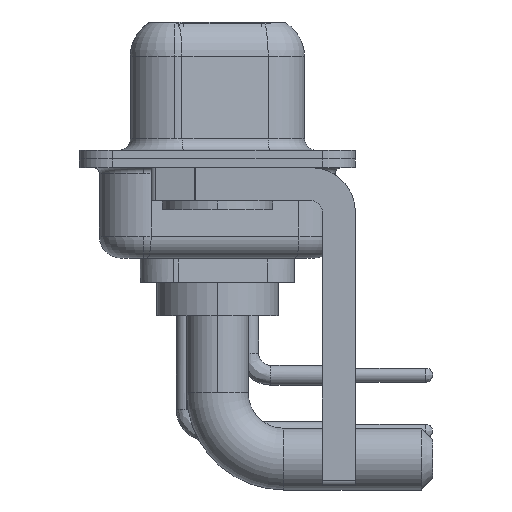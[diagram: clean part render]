
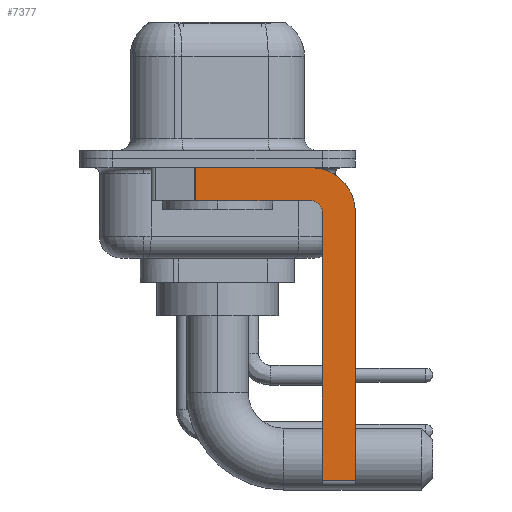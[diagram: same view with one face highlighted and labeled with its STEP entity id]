
A CAD part, left-side view. The second image highlights one B-rep face of the part: STEP entity #7377.
In plain terms, the highlighted planar face has unit normal (-1, 0, 0).
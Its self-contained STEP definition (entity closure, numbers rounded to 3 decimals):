
#596 = CIRCLE ( 'NONE', #11377, 0.5 ) ;
#609 = LINE ( 'NONE', #10292, #14014 ) ;
#762 = CARTESIAN_POINT ( 'NONE',  ( -2.9, -4.75, -2.4 ) ) ;
#1250 = CARTESIAN_POINT ( 'NONE',  ( -2.9, -4.25, -1.9 ) ) ;
#1425 = EDGE_CURVE ( 'NONE', #2869, #2047, #6243, .T. ) ;
#1938 = EDGE_CURVE ( 'NONE', #14677, #5587, #12662, .T. ) ;
#2047 = VERTEX_POINT ( 'NONE', #6836 ) ;
#2358 = EDGE_CURVE ( 'NONE', #2387, #14966, #5190, .T. ) ;
#2387 = VERTEX_POINT ( 'NONE', #14862 ) ;
#2869 = VERTEX_POINT ( 'NONE', #4990 ) ;
#3490 = EDGE_CURVE ( 'NONE', #2387, #14677, #17820, .T. ) ;
#3583 = EDGE_LOOP ( 'NONE', ( #13908, #8388, #13151, #5882, #15429, #6358, #17885, #15256 ) ) ;
#3808 = DIRECTION ( 'NONE',  ( 0., 0., 1. ) ) ;
#3945 = VECTOR ( 'NONE', #9134, 1000. ) ;
#4218 = EDGE_CURVE ( 'NONE', #5587, #2047, #9379, .T. ) ;
#4708 = VECTOR ( 'NONE', #3808, 1000. ) ;
#4990 = CARTESIAN_POINT ( 'NONE',  ( -2.9, -4.75, -14.55 ) ) ;
#5190 = LINE ( 'NONE', #15040, #3945 ) ;
#5485 = DIRECTION ( 'NONE',  ( 0., 0., -1. ) ) ;
#5587 = VERTEX_POINT ( 'NONE', #12764 ) ;
#5612 = EDGE_CURVE ( 'NONE', #2869, #15166, #12113, .T. ) ;
#5645 = CARTESIAN_POINT ( 'NONE',  ( -2.9, -4.25, -2.4 ) ) ;
#5686 = AXIS2_PLACEMENT_3D ( 'NONE', #14198, #7265, #6060 ) ;
#5882 = ORIENTED_EDGE ( 'NONE', *, *, #13888, .F. ) ;
#6060 = DIRECTION ( 'NONE',  ( 0., 0., -1. ) ) ;
#6243 = LINE ( 'NONE', #17651, #9725 ) ;
#6356 = CARTESIAN_POINT ( 'NONE',  ( -2.9, -4.75, -14.8 ) ) ;
#6358 = ORIENTED_EDGE ( 'NONE', *, *, #1425, .T. ) ;
#6836 = CARTESIAN_POINT ( 'NONE',  ( -2.9, -6.25, -14.55 ) ) ;
#7265 = DIRECTION ( 'NONE',  ( 1., 0., 0. ) ) ;
#7377 = ADVANCED_FACE ( 'NONE', ( #8645 ), #9012, .F. ) ;
#7472 = VECTOR ( 'NONE', #8072, 1000. ) ;
#7567 = VERTEX_POINT ( 'NONE', #1250 ) ;
#8072 = DIRECTION ( 'NONE',  ( 0., -1., 0. ) ) ;
#8346 = CARTESIAN_POINT ( 'NONE',  ( -2.9, 3., -0.4 ) ) ;
#8388 = ORIENTED_EDGE ( 'NONE', *, *, #2358, .T. ) ;
#8645 = FACE_OUTER_BOUND ( 'NONE', #3583, .T. ) ;
#9012 = PLANE ( 'NONE',  #5686 ) ;
#9134 = DIRECTION ( 'NONE',  ( 0., 0., -1. ) ) ;
#9379 = LINE ( 'NONE', #14931, #11698 ) ;
#9725 = VECTOR ( 'NONE', #11838, 1000. ) ;
#9873 = DIRECTION ( 'NONE',  ( 1., 0., 0. ) ) ;
#10292 = CARTESIAN_POINT ( 'NONE',  ( -2.9, -4.25, -1.9 ) ) ;
#10447 = CARTESIAN_POINT ( 'NONE',  ( -2.9, -4.25, -2.4 ) ) ;
#11377 = AXIS2_PLACEMENT_3D ( 'NONE', #10447, #11893, #15988 ) ;
#11698 = VECTOR ( 'NONE', #17758, 1000. ) ;
#11838 = DIRECTION ( 'NONE',  ( 0., -1., 0. ) ) ;
#11893 = DIRECTION ( 'NONE',  ( -1., 0., 0. ) ) ;
#12113 = LINE ( 'NONE', #6356, #4708 ) ;
#12662 = CIRCLE ( 'NONE', #13251, 2. ) ;
#12764 = CARTESIAN_POINT ( 'NONE',  ( -2.9, -6.25, -2.4 ) ) ;
#13151 = ORIENTED_EDGE ( 'NONE', *, *, #14746, .F. ) ;
#13251 = AXIS2_PLACEMENT_3D ( 'NONE', #5645, #9873, #5485 ) ;
#13888 = EDGE_CURVE ( 'NONE', #15166, #7567, #596, .T. ) ;
#13908 = ORIENTED_EDGE ( 'NONE', *, *, #3490, .F. ) ;
#14014 = VECTOR ( 'NONE', #14460, 1000. ) ;
#14196 = CARTESIAN_POINT ( 'NONE',  ( -2.9, -4.25, -0.4 ) ) ;
#14198 = CARTESIAN_POINT ( 'NONE',  ( -2.9, -4.25, -2.4 ) ) ;
#14460 = DIRECTION ( 'NONE',  ( 0., 1., 0. ) ) ;
#14677 = VERTEX_POINT ( 'NONE', #14196 ) ;
#14746 = EDGE_CURVE ( 'NONE', #7567, #14966, #609, .T. ) ;
#14862 = CARTESIAN_POINT ( 'NONE',  ( -2.9, 0.978, -0.4 ) ) ;
#14931 = CARTESIAN_POINT ( 'NONE',  ( -2.9, -6.25, -2.4 ) ) ;
#14966 = VERTEX_POINT ( 'NONE', #15538 ) ;
#15040 = CARTESIAN_POINT ( 'NONE',  ( -2.9, 0.978, -1.9 ) ) ;
#15166 = VERTEX_POINT ( 'NONE', #762 ) ;
#15256 = ORIENTED_EDGE ( 'NONE', *, *, #1938, .F. ) ;
#15429 = ORIENTED_EDGE ( 'NONE', *, *, #5612, .F. ) ;
#15538 = CARTESIAN_POINT ( 'NONE',  ( -2.9, 0.978, -1.9 ) ) ;
#15988 = DIRECTION ( 'NONE',  ( 0., 0., 1. ) ) ;
#17651 = CARTESIAN_POINT ( 'NONE',  ( -2.9, -4.25, -14.55 ) ) ;
#17758 = DIRECTION ( 'NONE',  ( 0., 0., -1. ) ) ;
#17820 = LINE ( 'NONE', #8346, #7472 ) ;
#17885 = ORIENTED_EDGE ( 'NONE', *, *, #4218, .F. ) ;
